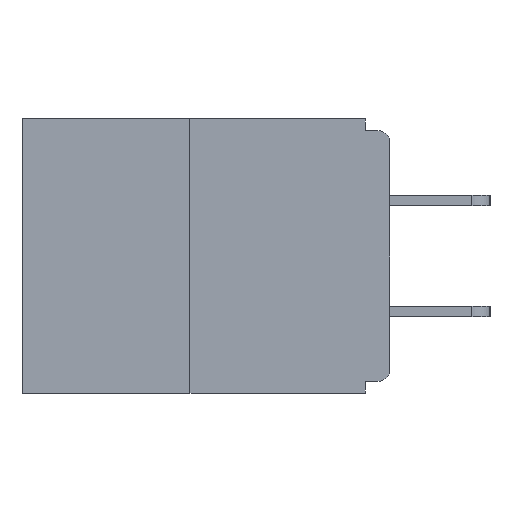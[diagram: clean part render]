
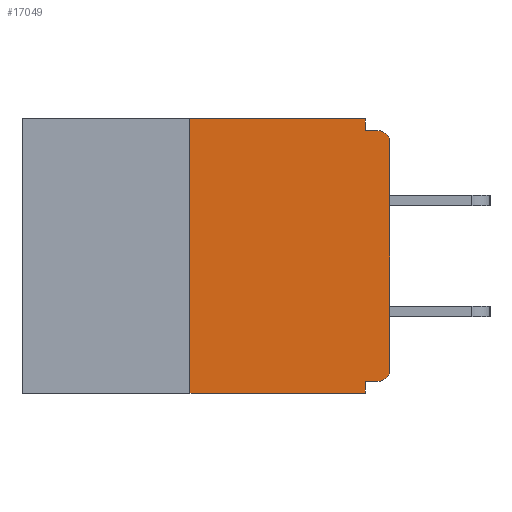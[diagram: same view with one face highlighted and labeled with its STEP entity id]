
A CAD part, left-side view. The second image highlights one B-rep face of the part: STEP entity #17049.
In plain terms, the highlighted planar face has unit normal (-1, 0, 0).
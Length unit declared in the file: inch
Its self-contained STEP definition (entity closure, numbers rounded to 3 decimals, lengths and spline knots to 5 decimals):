
#209 = VECTOR ( 'NONE', #1595, 39.37008 ) ;
#252 = VECTOR ( 'NONE', #16539, 39.37008 ) ;
#344 = ORIENTED_EDGE ( 'NONE', *, *, #6274, .T. ) ;
#455 = CARTESIAN_POINT ( 'NONE',  ( 0., 0.031, -0.343 ) ) ;
#982 = CIRCLE ( 'NONE', #26760, 0.015 ) ;
#1081 = ORIENTED_EDGE ( 'NONE', *, *, #10439, .T. ) ;
#1191 = VERTEX_POINT ( 'NONE', #15576 ) ;
#1497 = CARTESIAN_POINT ( 'NONE',  ( 0., 0.015, -0.015 ) ) ;
#1595 = DIRECTION ( 'NONE',  ( 0., -1., 0. ) ) ;
#2241 = EDGE_CURVE ( 'NONE', #24286, #11959, #9696, .T. ) ;
#2268 = EDGE_CURVE ( 'NONE', #11710, #20267, #982, .T. ) ;
#2664 = VERTEX_POINT ( 'NONE', #22492 ) ;
#3527 = CARTESIAN_POINT ( 'NONE',  ( 0., 0.46, 0. ) ) ;
#4557 = DIRECTION ( 'NONE',  ( 0., 0., -1. ) ) ;
#4662 = ORIENTED_EDGE ( 'NONE', *, *, #2268, .T. ) ;
#4989 = CARTESIAN_POINT ( 'NONE',  ( 0., 0., -0.313 ) ) ;
#5768 = DIRECTION ( 'NONE',  ( 0., 0., 1. ) ) ;
#5830 = VERTEX_POINT ( 'NONE', #19375 ) ;
#5857 = VECTOR ( 'NONE', #12301, 39.37008 ) ;
#6274 = EDGE_CURVE ( 'NONE', #5830, #19648, #16576, .T. ) ;
#6480 = LINE ( 'NONE', #14722, #13579 ) ;
#7199 = VECTOR ( 'NONE', #5768, 39.37008 ) ;
#7461 = LINE ( 'NONE', #23034, #252 ) ;
#7883 = CARTESIAN_POINT ( 'NONE',  ( 0., 0.015, -0.328 ) ) ;
#7889 = PLANE ( 'NONE',  #10392 ) ;
#8794 = EDGE_CURVE ( 'NONE', #1191, #20267, #12656, .T. ) ;
#8998 = CARTESIAN_POINT ( 'NONE',  ( 0., 0.031, -0.343 ) ) ;
#9696 = CIRCLE ( 'NONE', #21688, 0.015 ) ;
#9803 = LINE ( 'NONE', #20630, #7199 ) ;
#9843 = VECTOR ( 'NONE', #12100, 39.37008 ) ;
#10267 = DIRECTION ( 'NONE',  ( 0., 1., 0. ) ) ;
#10341 = DIRECTION ( 'NONE',  ( 0., 0., -1. ) ) ;
#10392 = AXIS2_PLACEMENT_3D ( 'NONE', #18990, #23596, #10341 ) ;
#10439 = EDGE_CURVE ( 'NONE', #11959, #11710, #7461, .T. ) ;
#10558 = EDGE_LOOP ( 'NONE', ( #13371, #22045, #344, #17559, #27508, #24088, #1081, #4662, #19393, #18198 ) ) ;
#11635 = DIRECTION ( 'NONE',  ( 0., 0., -1. ) ) ;
#11710 = VERTEX_POINT ( 'NONE', #25233 ) ;
#11824 = DIRECTION ( 'NONE',  ( -1., 0., 0. ) ) ;
#11959 = VERTEX_POINT ( 'NONE', #4989 ) ;
#12100 = DIRECTION ( 'NONE',  ( 0., -1., 0. ) ) ;
#12301 = DIRECTION ( 'NONE',  ( 0., -1., 0. ) ) ;
#12656 = LINE ( 'NONE', #16991, #209 ) ;
#12866 = DIRECTION ( 'NONE',  ( 0., 0., -1. ) ) ;
#13353 = CARTESIAN_POINT ( 'NONE',  ( 0., 0.031, -0.328 ) ) ;
#13371 = ORIENTED_EDGE ( 'NONE', *, *, #18713, .F. ) ;
#13579 = VECTOR ( 'NONE', #10267, 39.37008 ) ;
#13747 = VERTEX_POINT ( 'NONE', #13353 ) ;
#14706 = CARTESIAN_POINT ( 'NONE',  ( 0., 0.46, -0.343 ) ) ;
#14722 = CARTESIAN_POINT ( 'NONE',  ( 0., 0., -0.328 ) ) ;
#14766 = DIRECTION ( 'NONE',  ( -1., 0., 0. ) ) ;
#15336 = CARTESIAN_POINT ( 'NONE',  ( 0., 0.031, 0. ) ) ;
#15426 = VECTOR ( 'NONE', #11635, 39.37008 ) ;
#15576 = CARTESIAN_POINT ( 'NONE',  ( 0., 0.031, -0.015 ) ) ;
#16539 = DIRECTION ( 'NONE',  ( 0., 0., 1. ) ) ;
#16576 = LINE ( 'NONE', #14706, #9843 ) ;
#16799 = EDGE_CURVE ( 'NONE', #24286, #13747, #6480, .T. ) ;
#16991 = CARTESIAN_POINT ( 'NONE',  ( 0., 0., -0.015 ) ) ;
#17049 = ADVANCED_FACE ( 'NONE', ( #23158 ), #7889, .F. ) ;
#17506 = CARTESIAN_POINT ( 'NONE',  ( 0., 0.015, -0.313 ) ) ;
#17559 = ORIENTED_EDGE ( 'NONE', *, *, #27751, .F. ) ;
#18198 = ORIENTED_EDGE ( 'NONE', *, *, #27166, .F. ) ;
#18366 = EDGE_CURVE ( 'NONE', #5830, #2664, #9803, .T. ) ;
#18713 = EDGE_CURVE ( 'NONE', #2664, #28068, #23253, .T. ) ;
#18990 = CARTESIAN_POINT ( 'NONE',  ( 0., 0.46, 0. ) ) ;
#19375 = CARTESIAN_POINT ( 'NONE',  ( 0., 0.25, -0.343 ) ) ;
#19393 = ORIENTED_EDGE ( 'NONE', *, *, #8794, .F. ) ;
#19648 = VERTEX_POINT ( 'NONE', #8998 ) ;
#20267 = VERTEX_POINT ( 'NONE', #1497 ) ;
#20630 = CARTESIAN_POINT ( 'NONE',  ( 0., 0.25, 0. ) ) ;
#21673 = LINE ( 'NONE', #24114, #25554 ) ;
#21688 = AXIS2_PLACEMENT_3D ( 'NONE', #17506, #14766, #28093 ) ;
#22045 = ORIENTED_EDGE ( 'NONE', *, *, #18366, .F. ) ;
#22205 = LINE ( 'NONE', #455, #15426 ) ;
#22492 = CARTESIAN_POINT ( 'NONE',  ( 0., 0.25, 0. ) ) ;
#23034 = CARTESIAN_POINT ( 'NONE',  ( 0., 0., 0. ) ) ;
#23158 = FACE_OUTER_BOUND ( 'NONE', #10558, .T. ) ;
#23253 = LINE ( 'NONE', #3527, #5857 ) ;
#23596 = DIRECTION ( 'NONE',  ( 1., 0., 0. ) ) ;
#24088 = ORIENTED_EDGE ( 'NONE', *, *, #2241, .T. ) ;
#24114 = CARTESIAN_POINT ( 'NONE',  ( 0., 0.031, 0. ) ) ;
#24286 = VERTEX_POINT ( 'NONE', #7883 ) ;
#25233 = CARTESIAN_POINT ( 'NONE',  ( 0., 0., -0.03 ) ) ;
#25554 = VECTOR ( 'NONE', #12866, 39.37008 ) ;
#26760 = AXIS2_PLACEMENT_3D ( 'NONE', #27143, #11824, #4557 ) ;
#27143 = CARTESIAN_POINT ( 'NONE',  ( 0., 0.015, -0.03 ) ) ;
#27166 = EDGE_CURVE ( 'NONE', #28068, #1191, #21673, .T. ) ;
#27508 = ORIENTED_EDGE ( 'NONE', *, *, #16799, .F. ) ;
#27751 = EDGE_CURVE ( 'NONE', #13747, #19648, #22205, .T. ) ;
#28068 = VERTEX_POINT ( 'NONE', #15336 ) ;
#28093 = DIRECTION ( 'NONE',  ( 0., 0., -1. ) ) ;
